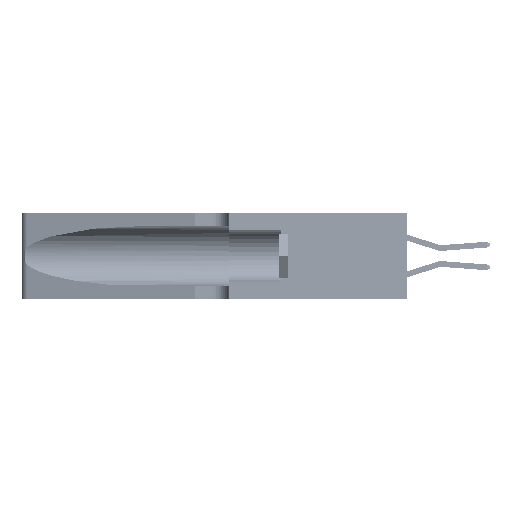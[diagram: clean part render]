
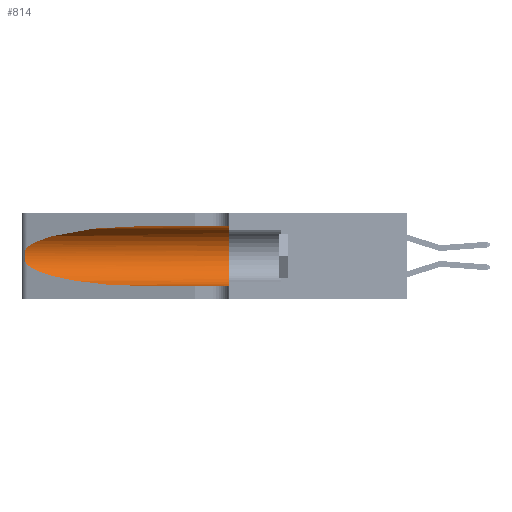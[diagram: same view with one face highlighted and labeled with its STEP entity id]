
A CAD part, left-side view. The second image highlights one B-rep face of the part: STEP entity #814.
In plain terms, the highlighted cylindrical face has radius 3.308 mm (diameter 6.617 mm), a partial arc.
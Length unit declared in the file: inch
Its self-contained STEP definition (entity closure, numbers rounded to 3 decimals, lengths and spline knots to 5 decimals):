
#169 = CARTESIAN_POINT ( 'NONE',  ( 0.25555, 1.22993, 0.14849 ) ) ;
#322 = CARTESIAN_POINT ( 'NONE',  ( 0.25487, 1.22718, 0.14631 ) ) ;
#656 = CARTESIAN_POINT ( 'NONE',  ( 0.25856, 1.23593, 0.16098 ) ) ;
#796 = CARTESIAN_POINT ( 'NONE',  ( 0.1305, 0.35, 0.05475 ) ) ;
#814 = ADVANCED_FACE ( 'NONE', ( #6429 ), #32647, .F. ) ;
#3405 = CARTESIAN_POINT ( 'NONE',  ( 0.2373, 1.15595, 0.08982 ) ) ;
#4124 = CARTESIAN_POINT ( 'NONE',  ( 0.25787, 1.23484, 0.2124 ) ) ;
#5156 = VECTOR ( 'NONE', #7390, 39.37008 ) ;
#6009 = CARTESIAN_POINT ( 'NONE',  ( 0.18966, 0.96281, 0.31525 ) ) ;
#6429 = FACE_OUTER_BOUND ( 'NONE', #20511, .T. ) ;
#6456 = VERTEX_POINT ( 'NONE', #31257 ) ;
#6634 = CARTESIAN_POINT ( 'NONE',  ( 0.2373, 1.15595, 0.28018 ) ) ;
#6694 = ORIENTED_EDGE ( 'NONE', *, *, #9804, .T. ) ;
#7390 = DIRECTION ( 'NONE',  ( 0., -1., 0. ) ) ;
#9018 =( BOUNDED_CURVE ( )  B_SPLINE_CURVE ( 3, ( #9986, #6009, #6634, #31475 ),
 .UNSPECIFIED., .F., .T. ) 
 B_SPLINE_CURVE_WITH_KNOTS ( ( 4, 4 ),
 ( 1.5708, 2.84003 ),
 .UNSPECIFIED. ) 
 CURVE ( )  GEOMETRIC_REPRESENTATION_ITEM ( )  RATIONAL_B_SPLINE_CURVE ( ( 1., 0.87, 0.87, 1. ) ) 
 REPRESENTATION_ITEM ( '' )  );
#9804 = EDGE_CURVE ( 'NONE', #38107, #16051, #27971, .T. ) ;
#9986 = CARTESIAN_POINT ( 'NONE',  ( 0.1305, 0.72297, 0.31525 ) ) ;
#10641 = VERTEX_POINT ( 'NONE', #796 ) ;
#10961 = CARTESIAN_POINT ( 'NONE',  ( 0.25555, 1.22994, 0.2215 ) ) ;
#11358 = EDGE_CURVE ( 'NONE', #39433, #38107, #20986, .T. ) ;
#12687 = DIRECTION ( 'NONE',  ( 0., 0., 1. ) ) ;
#13036 = CARTESIAN_POINT ( 'NONE',  ( 0.1305, 1.61858, 0.31525 ) ) ;
#13039 = CARTESIAN_POINT ( 'NONE',  ( 0.25487, 1.22718, 0.22369 ) ) ;
#13075 = VECTOR ( 'NONE', #39116, 39.37008 ) ;
#13592 = ORIENTED_EDGE ( 'NONE', *, *, #21655, .F. ) ;
#14753 = CARTESIAN_POINT ( 'NONE',  ( 0.25854, 1.2359, 0.20912 ) ) ;
#15057 = CARTESIAN_POINT ( 'NONE',  ( 0.26018, 1.23835, 0.19895 ) ) ;
#16051 = VERTEX_POINT ( 'NONE', #24879 ) ;
#18197 = ORIENTED_EDGE ( 'NONE', *, *, #22345, .T. ) ;
#18292 = CARTESIAN_POINT ( 'NONE',  ( 0.26017, 1.23833, 0.17102 ) ) ;
#18836 = CARTESIAN_POINT ( 'NONE',  ( 0.1305, 1.61858, 0.185 ) ) ;
#20511 = EDGE_LOOP ( 'NONE', ( #18197, #42954, #6694, #34593, #24099, #13592 ) ) ;
#20986 = B_SPLINE_CURVE_WITH_KNOTS ( 'NONE', 3,
 ( #22422, #10961, #36890, #4124, #14753, #15057, #29566, #22116, #18292, #656, #40511, #44148, #169, #322 ),
 .UNSPECIFIED., .F., .F.,
 ( 4, 2, 2, 2, 2, 2, 4 ),
 ( 0., 0.00027, 0.00053, 0.00107, 0.0016, 0.00187, 0.00214 ),
 .UNSPECIFIED. ) ;
#21655 = EDGE_CURVE ( 'NONE', #40112, #6456, #41466, .T. ) ;
#22116 = CARTESIAN_POINT ( 'NONE',  ( 0.26075, 1.23896, 0.178 ) ) ;
#22345 = EDGE_CURVE ( 'NONE', #40112, #39433, #9018, .T. ) ;
#22422 = CARTESIAN_POINT ( 'NONE',  ( 0.25487, 1.22718, 0.22369 ) ) ;
#23353 = CARTESIAN_POINT ( 'NONE',  ( 0.1305, 0.72297, 0.31525 ) ) ;
#23523 = CARTESIAN_POINT ( 'NONE',  ( 0.1305, 0.35, 0.185 ) ) ;
#24099 = ORIENTED_EDGE ( 'NONE', *, *, #31469, .F. ) ;
#24879 = CARTESIAN_POINT ( 'NONE',  ( 0.1305, 0.72297, 0.05475 ) ) ;
#26283 = DIRECTION ( 'NONE',  ( 0., -1., 0. ) ) ;
#27971 =( BOUNDED_CURVE ( )  B_SPLINE_CURVE ( 3, ( #28514, #3405, #42925, #36005 ),
 .UNSPECIFIED., .F., .F. ) 
 B_SPLINE_CURVE_WITH_KNOTS ( ( 4, 4 ),
 ( 3.44316, 4.71239 ),
 .UNSPECIFIED. ) 
 CURVE ( )  GEOMETRIC_REPRESENTATION_ITEM ( )  RATIONAL_B_SPLINE_CURVE ( ( 1., 0.87, 0.87, 1. ) ) 
 REPRESENTATION_ITEM ( '' )  );
#28514 = CARTESIAN_POINT ( 'NONE',  ( 0.25487, 1.22718, 0.14631 ) ) ;
#29566 = CARTESIAN_POINT ( 'NONE',  ( 0.26075, 1.23896, 0.19203 ) ) ;
#29639 = DIRECTION ( 'NONE',  ( 0., 0., -1. ) ) ;
#31257 = CARTESIAN_POINT ( 'NONE',  ( 0.1305, 0.35, 0.31525 ) ) ;
#31469 = EDGE_CURVE ( 'NONE', #6456, #10641, #40686, .T. ) ;
#31475 = CARTESIAN_POINT ( 'NONE',  ( 0.25487, 1.22718, 0.22369 ) ) ;
#31994 = CARTESIAN_POINT ( 'NONE',  ( 0.25487, 1.22718, 0.14631 ) ) ;
#32647 = CYLINDRICAL_SURFACE ( 'NONE', #39216, 0.13025 ) ;
#34593 = ORIENTED_EDGE ( 'NONE', *, *, #44488, .T. ) ;
#36005 = CARTESIAN_POINT ( 'NONE',  ( 0.1305, 0.72297, 0.05475 ) ) ;
#36890 = CARTESIAN_POINT ( 'NONE',  ( 0.25639, 1.23184, 0.21858 ) ) ;
#38107 = VERTEX_POINT ( 'NONE', #31994 ) ;
#39116 = DIRECTION ( 'NONE',  ( 0., -1., 0. ) ) ;
#39216 = AXIS2_PLACEMENT_3D ( 'NONE', #18836, #26283, #29639 ) ;
#39433 = VERTEX_POINT ( 'NONE', #13039 ) ;
#40112 = VERTEX_POINT ( 'NONE', #23353 ) ;
#40511 = CARTESIAN_POINT ( 'NONE',  ( 0.25789, 1.23486, 0.15765 ) ) ;
#40686 = CIRCLE ( 'NONE', #42214, 0.13025 ) ;
#41441 = DIRECTION ( 'NONE',  ( 0., 1., 0. ) ) ;
#41466 = LINE ( 'NONE', #13036, #13075 ) ;
#42214 = AXIS2_PLACEMENT_3D ( 'NONE', #23523, #41441, #12687 ) ;
#42787 = CARTESIAN_POINT ( 'NONE',  ( 0.1305, 1.61858, 0.05475 ) ) ;
#42925 = CARTESIAN_POINT ( 'NONE',  ( 0.18966, 0.96281, 0.05475 ) ) ;
#42954 = ORIENTED_EDGE ( 'NONE', *, *, #11358, .T. ) ;
#43842 = LINE ( 'NONE', #42787, #5156 ) ;
#44148 = CARTESIAN_POINT ( 'NONE',  ( 0.25639, 1.23186, 0.15144 ) ) ;
#44488 = EDGE_CURVE ( 'NONE', #16051, #10641, #43842, .T. ) ;
